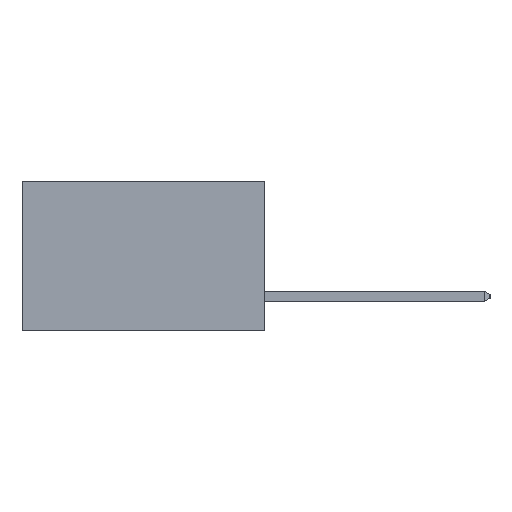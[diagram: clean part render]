
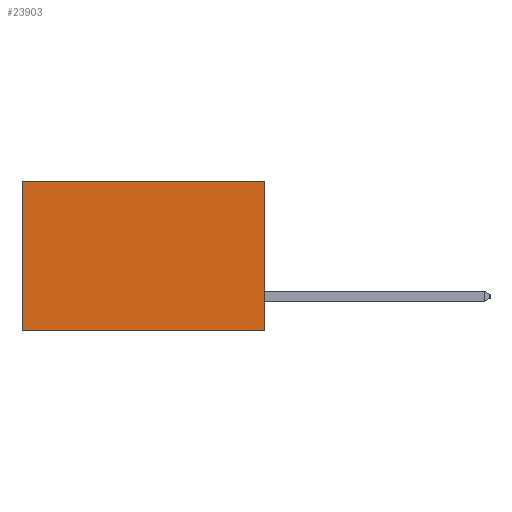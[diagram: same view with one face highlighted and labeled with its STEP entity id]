
A CAD part, left-side view. The second image highlights one B-rep face of the part: STEP entity #23903.
In plain terms, the highlighted planar face has unit normal (-1, 0, 0).
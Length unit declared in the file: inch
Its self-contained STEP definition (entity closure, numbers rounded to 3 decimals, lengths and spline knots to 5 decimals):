
#661 = VECTOR ( 'NONE', #21647, 39.37008 ) ;
#1568 = CARTESIAN_POINT ( 'NONE',  ( 0.2615, 0., 0. ) ) ;
#2741 = AXIS2_PLACEMENT_3D ( 'NONE', #19590, #9867, #23499 ) ;
#3181 = FACE_OUTER_BOUND ( 'NONE', #3751, .T. ) ;
#3487 = VERTEX_POINT ( 'NONE', #13146 ) ;
#3751 = EDGE_LOOP ( 'NONE', ( #15353, #6136, #15489, #17763 ) ) ;
#5414 = EDGE_CURVE ( 'NONE', #17688, #5440, #21821, .T. ) ;
#5440 = VERTEX_POINT ( 'NONE', #5752 ) ;
#5752 = CARTESIAN_POINT ( 'NONE',  ( 0.2615, 0.6, -0.37 ) ) ;
#5937 = EDGE_CURVE ( 'NONE', #15260, #5440, #20579, .T. ) ;
#5974 = LINE ( 'NONE', #19708, #661 ) ;
#6136 = ORIENTED_EDGE ( 'NONE', *, *, #5937, .F. ) ;
#9613 = VECTOR ( 'NONE', #12736, 39.37008 ) ;
#9867 = DIRECTION ( 'NONE',  ( 1., 0., 0. ) ) ;
#11940 = VECTOR ( 'NONE', #15365, 39.37008 ) ;
#11977 = CARTESIAN_POINT ( 'NONE',  ( 0.2615, 0.6, -0.37 ) ) ;
#12736 = DIRECTION ( 'NONE',  ( 0., 1., 0. ) ) ;
#13146 = CARTESIAN_POINT ( 'NONE',  ( 0.2615, 0., 0. ) ) ;
#13355 = CARTESIAN_POINT ( 'NONE',  ( 0.2615, 0., -0.37 ) ) ;
#13871 = DIRECTION ( 'NONE',  ( 0., 0., -1. ) ) ;
#15260 = VERTEX_POINT ( 'NONE', #22979 ) ;
#15353 = ORIENTED_EDGE ( 'NONE', *, *, #5414, .T. ) ;
#15365 = DIRECTION ( 'NONE',  ( 0., 1., 0. ) ) ;
#15489 = ORIENTED_EDGE ( 'NONE', *, *, #17449, .F. ) ;
#15885 = EDGE_CURVE ( 'NONE', #3487, #17688, #17221, .T. ) ;
#16680 = VECTOR ( 'NONE', #13871, 39.37008 ) ;
#17221 = LINE ( 'NONE', #1568, #11940 ) ;
#17449 = EDGE_CURVE ( 'NONE', #3487, #15260, #5974, .T. ) ;
#17688 = VERTEX_POINT ( 'NONE', #22232 ) ;
#17763 = ORIENTED_EDGE ( 'NONE', *, *, #15885, .T. ) ;
#19590 = CARTESIAN_POINT ( 'NONE',  ( 0.2615, 0., -0.37 ) ) ;
#19708 = CARTESIAN_POINT ( 'NONE',  ( 0.2615, 0., -0.37 ) ) ;
#20579 = LINE ( 'NONE', #13355, #9613 ) ;
#21516 = PLANE ( 'NONE',  #2741 ) ;
#21647 = DIRECTION ( 'NONE',  ( 0., 0., -1. ) ) ;
#21821 = LINE ( 'NONE', #11977, #16680 ) ;
#22232 = CARTESIAN_POINT ( 'NONE',  ( 0.2615, 0.6, 0. ) ) ;
#22979 = CARTESIAN_POINT ( 'NONE',  ( 0.2615, 0., -0.37 ) ) ;
#23499 = DIRECTION ( 'NONE',  ( 0., 0., -1. ) ) ;
#23903 = ADVANCED_FACE ( 'NONE', ( #3181 ), #21516, .F. ) ;
